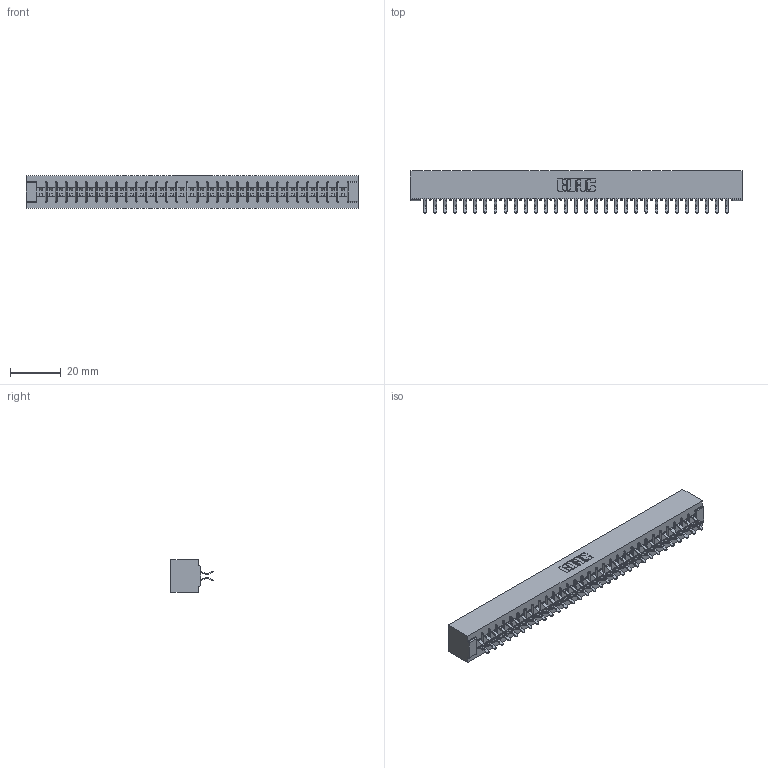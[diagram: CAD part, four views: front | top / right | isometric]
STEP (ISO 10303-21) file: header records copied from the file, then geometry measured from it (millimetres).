
FILE_DESCRIPTION (( 'STEP AP203' ), '1' );
FILE_NAME ('315-062-556-201.STEP', '2019-09-10T20:22:06', ( '' ), ( '' ), 'SwSTEP 2.0', 'SolidWorks 2016', '' );
FILE_SCHEMA (( 'CONFIG_CONTROL_DESIGN' ));
Length unit declared in the file: inch
Products named in the file (3): 305 Part_No Mounting; 305-290-001_556; 315-062-556-201
Assembly tree (63 placements, depth 2):
  315-062-556-201
    305 Part_No Mounting
    305-290-001_556  x62
Bounding box: 130.71 x 16.64 x 12.7 mm (x, y, z)
Volume: 14048.9 mm3; surface area: 18039.2 mm2
Topology: 63 solids, 63 shells, 3580 faces, 10305 edges, 6702 vertices
Faces by surface type: plane 1986, cylinder 1470, sphere 124
Entity records: 34848 total; most frequent: CARTESIAN_POINT 5767, ORIENTED_EDGE 5722, DIRECTION 5589, EDGE_CURVE 2861, VECTOR 2301, LINE 2301, VERTEX_POINT 1822, AXIS2_PLACEMENT_3D 1644
